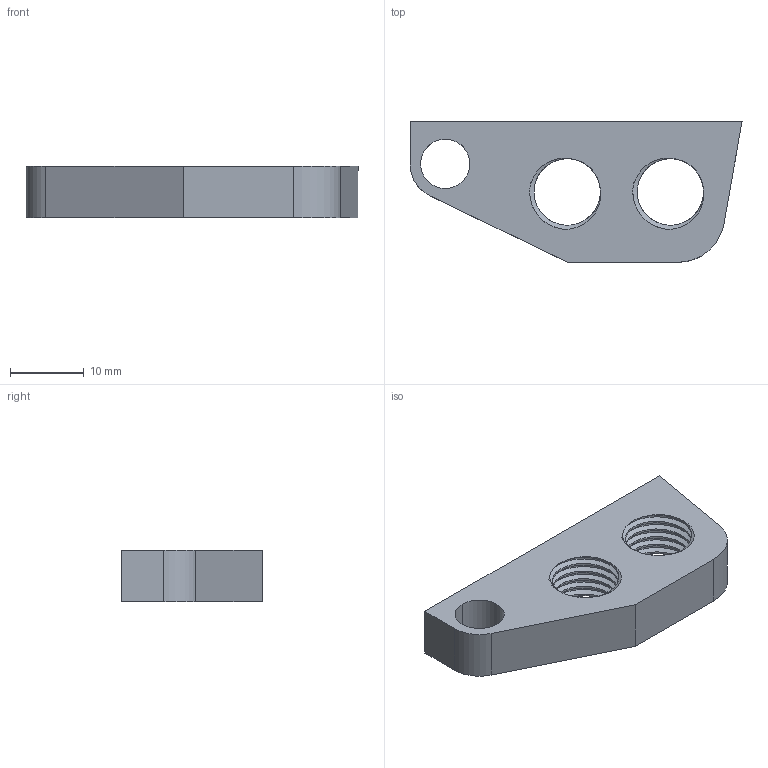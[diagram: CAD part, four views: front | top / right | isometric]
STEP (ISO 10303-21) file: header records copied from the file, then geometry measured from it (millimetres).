
FILE_DESCRIPTION (( 'STEP AP203' ), '1' );
FILE_NAME ('AF-WF-LR-PRT-003-STEP.STEP', '2020-07-21T18:18:29', ( '' ), ( '' ), 'SwSTEP 2.0', 'SolidWorks 2018', '' );
FILE_SCHEMA (( 'CONFIG_CONTROL_DESIGN' ));
Length unit declared in the file: inch
Products named in the file (1): AF-WF-LR-PRT-003-STEP
Bounding box: 44.97 x 19.05 x 6.91 mm (x, y, z)
Volume: 3637.3 mm3; surface area: 2624.2 mm2
Topology: 1 solids, 1 shells, 41 faces, 117 edges, 78 vertices
Faces by surface type: cylinder 28, plane 7, bspline 6
Entity records: 3644 total; most frequent: CARTESIAN_POINT 2663, ORIENTED_EDGE 234, DIRECTION 141, EDGE_CURVE 117, VERTEX_POINT 78, AXIS2_PLACEMENT_3D 50, EDGE_LOOP 47, ADVANCED_FACE 41
